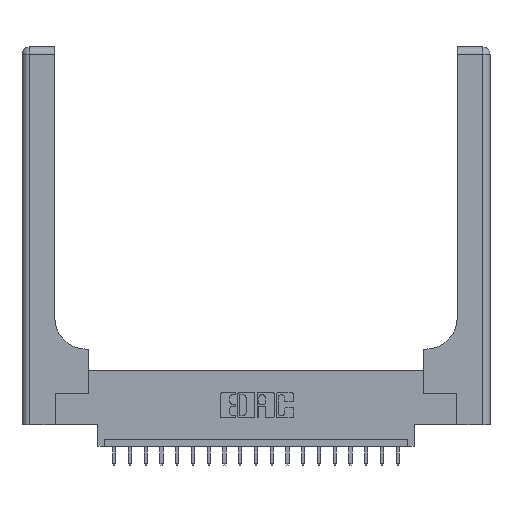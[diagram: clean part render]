
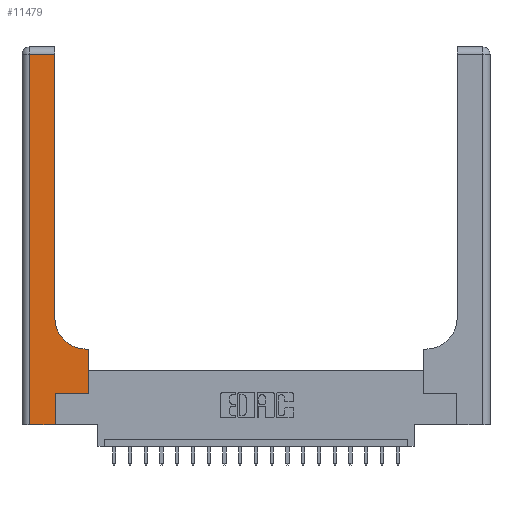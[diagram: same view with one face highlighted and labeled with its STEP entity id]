
A CAD part, top view. The second image highlights one B-rep face of the part: STEP entity #11479.
In plain terms, the highlighted planar face has unit normal (0, 0, 1).
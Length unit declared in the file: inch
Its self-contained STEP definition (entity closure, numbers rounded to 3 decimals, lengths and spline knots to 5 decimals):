
#1340 = ORIENTED_EDGE ( 'NONE', *, *, #18836, .T. ) ;
#1449 = CARTESIAN_POINT ( 'NONE',  ( 0., 0., 0.37 ) ) ;
#1571 = CARTESIAN_POINT ( 'NONE',  ( 0.26, 0.6, 0.37 ) ) ;
#1758 = CARTESIAN_POINT ( 'NONE',  ( 0.528, 0.25, 0.37 ) ) ;
#1869 = DIRECTION ( 'NONE',  ( 0., 0., -1. ) ) ;
#2005 = CARTESIAN_POINT ( 'NONE',  ( 0.265, 0.25, 0.37 ) ) ;
#2629 = EDGE_CURVE ( 'NONE', #2986, #9519, #9355, .T. ) ;
#2752 = DIRECTION ( 'NONE',  ( 0., 1., 0. ) ) ;
#2847 = DIRECTION ( 'NONE',  ( 0., 1., 0. ) ) ;
#2924 = CARTESIAN_POINT ( 'NONE',  ( 0., 3., 0.37 ) ) ;
#2986 = VERTEX_POINT ( 'NONE', #4587 ) ;
#3062 = CARTESIAN_POINT ( 'NONE',  ( 0.528, 0.6, 0.37 ) ) ;
#3333 = CARTESIAN_POINT ( 'NONE',  ( 0.51, 0.85, 0.37 ) ) ;
#4138 = VERTEX_POINT ( 'NONE', #1758 ) ;
#4176 = EDGE_CURVE ( 'NONE', #8449, #2986, #11522, .T. ) ;
#4587 = CARTESIAN_POINT ( 'NONE',  ( 0.26, 0.85, 0.37 ) ) ;
#4681 = VERTEX_POINT ( 'NONE', #3062 ) ;
#5065 = DIRECTION ( 'NONE',  ( 1., 0., 0. ) ) ;
#5289 = LINE ( 'NONE', #6562, #18019 ) ;
#5530 = AXIS2_PLACEMENT_3D ( 'NONE', #3333, #1869, #11136 ) ;
#5767 = LINE ( 'NONE', #6416, #19938 ) ;
#5897 = VECTOR ( 'NONE', #5065, 39.37008 ) ;
#6047 = VECTOR ( 'NONE', #2752, 39.37008 ) ;
#6164 = VERTEX_POINT ( 'NONE', #9479 ) ;
#6416 = CARTESIAN_POINT ( 'NONE',  ( 0., 2.94, 0.37 ) ) ;
#6512 = CARTESIAN_POINT ( 'NONE',  ( 0.265, 0., 0.37 ) ) ;
#6553 = ORIENTED_EDGE ( 'NONE', *, *, #14035, .T. ) ;
#6562 = CARTESIAN_POINT ( 'NONE',  ( 0.06, 3., 0.37 ) ) ;
#6699 = CARTESIAN_POINT ( 'NONE',  ( 0.06, 2.94, 0.37 ) ) ;
#7164 = CARTESIAN_POINT ( 'NONE',  ( 0.51, 0.6, 0.37 ) ) ;
#7435 = PLANE ( 'NONE',  #18685 ) ;
#7713 = CARTESIAN_POINT ( 'NONE',  ( 0.26, 3., 0.37 ) ) ;
#7960 = ORIENTED_EDGE ( 'NONE', *, *, #10403, .T. ) ;
#8449 = VERTEX_POINT ( 'NONE', #7164 ) ;
#8718 = LINE ( 'NONE', #8888, #6047 ) ;
#8803 = LINE ( 'NONE', #1449, #5897 ) ;
#8888 = CARTESIAN_POINT ( 'NONE',  ( 0.528, 0.25, 0.37 ) ) ;
#9156 = EDGE_CURVE ( 'NONE', #9519, #15045, #5767, .T. ) ;
#9213 = EDGE_CURVE ( 'NONE', #15045, #16293, #5289, .T. ) ;
#9226 = ORIENTED_EDGE ( 'NONE', *, *, #9156, .T. ) ;
#9355 = LINE ( 'NONE', #7713, #13788 ) ;
#9479 = CARTESIAN_POINT ( 'NONE',  ( 0.265, 0., 0.37 ) ) ;
#9519 = VERTEX_POINT ( 'NONE', #12632 ) ;
#9879 = DIRECTION ( 'NONE',  ( 1., 0., 0. ) ) ;
#10352 = LINE ( 'NONE', #6512, #19183 ) ;
#10403 = EDGE_CURVE ( 'NONE', #6164, #18835, #10352, .T. ) ;
#11107 = DIRECTION ( 'NONE',  ( -1., 0., 0. ) ) ;
#11136 = DIRECTION ( 'NONE',  ( 1., 0., 0. ) ) ;
#11479 = ADVANCED_FACE ( 'NONE', ( #14978 ), #7435, .F. ) ;
#11522 = CIRCLE ( 'NONE', #5530, 0.25 ) ;
#11688 = EDGE_CURVE ( 'NONE', #4681, #8449, #17426, .T. ) ;
#12530 = DIRECTION ( 'NONE',  ( -1., 0., 0. ) ) ;
#12632 = CARTESIAN_POINT ( 'NONE',  ( 0.26, 2.94, 0.37 ) ) ;
#13710 = ORIENTED_EDGE ( 'NONE', *, *, #11688, .T. ) ;
#13788 = VECTOR ( 'NONE', #2847, 39.37008 ) ;
#13852 = DIRECTION ( 'NONE',  ( -1., 0., 0. ) ) ;
#14035 = EDGE_CURVE ( 'NONE', #4138, #4681, #8718, .T. ) ;
#14331 = EDGE_LOOP ( 'NONE', ( #20188, #9226, #16956, #16922, #7960, #1340, #6553, #13710, #19576 ) ) ;
#14978 = FACE_OUTER_BOUND ( 'NONE', #14331, .T. ) ;
#15045 = VERTEX_POINT ( 'NONE', #6699 ) ;
#15129 = DIRECTION ( 'NONE',  ( 0., -1., 0. ) ) ;
#15934 = LINE ( 'NONE', #19353, #19594 ) ;
#16041 = CARTESIAN_POINT ( 'NONE',  ( 0.06, 0., 0.37 ) ) ;
#16293 = VERTEX_POINT ( 'NONE', #16041 ) ;
#16922 = ORIENTED_EDGE ( 'NONE', *, *, #18713, .T. ) ;
#16928 = VECTOR ( 'NONE', #11107, 39.37008 ) ;
#16956 = ORIENTED_EDGE ( 'NONE', *, *, #9213, .T. ) ;
#17148 = DIRECTION ( 'NONE',  ( 0., 0., -1. ) ) ;
#17426 = LINE ( 'NONE', #1571, #16928 ) ;
#17771 = DIRECTION ( 'NONE',  ( 0., 1., 0. ) ) ;
#18019 = VECTOR ( 'NONE', #15129, 39.37008 ) ;
#18685 = AXIS2_PLACEMENT_3D ( 'NONE', #2924, #17148, #13852 ) ;
#18713 = EDGE_CURVE ( 'NONE', #16293, #6164, #8803, .T. ) ;
#18835 = VERTEX_POINT ( 'NONE', #2005 ) ;
#18836 = EDGE_CURVE ( 'NONE', #18835, #4138, #15934, .T. ) ;
#19183 = VECTOR ( 'NONE', #17771, 39.37008 ) ;
#19353 = CARTESIAN_POINT ( 'NONE',  ( 0.265, 0.25, 0.37 ) ) ;
#19576 = ORIENTED_EDGE ( 'NONE', *, *, #4176, .T. ) ;
#19594 = VECTOR ( 'NONE', #9879, 39.37008 ) ;
#19938 = VECTOR ( 'NONE', #12530, 39.37008 ) ;
#20188 = ORIENTED_EDGE ( 'NONE', *, *, #2629, .T. ) ;
